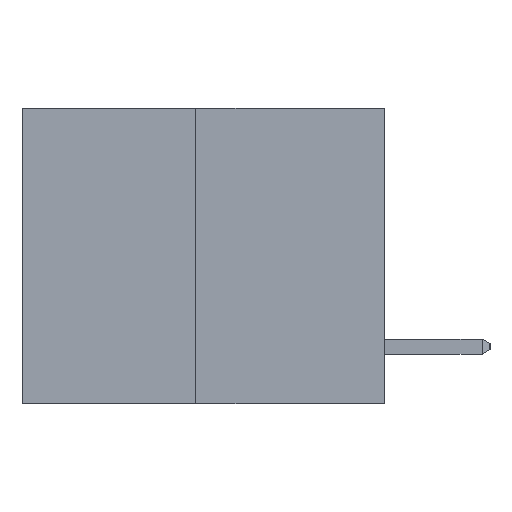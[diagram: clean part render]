
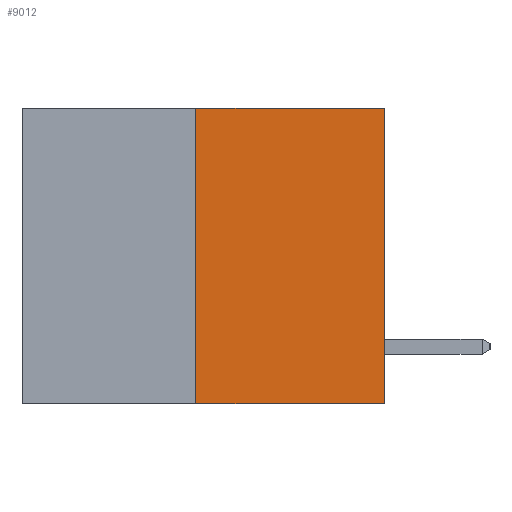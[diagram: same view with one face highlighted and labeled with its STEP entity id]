
A CAD part, left-side view. The second image highlights one B-rep face of the part: STEP entity #9012.
In plain terms, the highlighted planar face has unit normal (-1, 0, 0).
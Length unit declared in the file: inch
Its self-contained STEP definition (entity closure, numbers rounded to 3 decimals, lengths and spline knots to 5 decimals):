
#842 = EDGE_CURVE ( 'NONE', #2512, #4232, #8939, .T. ) ;
#925 = DIRECTION ( 'NONE',  ( 0., 0., 1. ) ) ;
#1031 = LINE ( 'NONE', #9667, #9418 ) ;
#1515 = CARTESIAN_POINT ( 'NONE',  ( 0., 0.312, 0. ) ) ;
#1947 = DIRECTION ( 'NONE',  ( 1., 0., 0. ) ) ;
#2512 = VERTEX_POINT ( 'NONE', #1515 ) ;
#2527 = ORIENTED_EDGE ( 'NONE', *, *, #4986, .F. ) ;
#2690 = CARTESIAN_POINT ( 'NONE',  ( 0., 0.6, -0.49 ) ) ;
#2900 = VECTOR ( 'NONE', #3539, 39.37008 ) ;
#3066 = ORIENTED_EDGE ( 'NONE', *, *, #842, .F. ) ;
#3245 = EDGE_CURVE ( 'NONE', #5120, #5028, #6477, .T. ) ;
#3539 = DIRECTION ( 'NONE',  ( 0., -1., 0. ) ) ;
#3736 = CARTESIAN_POINT ( 'NONE',  ( 0., 0., 0. ) ) ;
#3837 = ORIENTED_EDGE ( 'NONE', *, *, #8749, .T. ) ;
#3982 = VECTOR ( 'NONE', #925, 39.37008 ) ;
#4232 = VERTEX_POINT ( 'NONE', #3736 ) ;
#4310 = ORIENTED_EDGE ( 'NONE', *, *, #3245, .T. ) ;
#4333 = DIRECTION ( 'NONE',  ( 0., -1., 0. ) ) ;
#4986 = EDGE_CURVE ( 'NONE', #5120, #2512, #1031, .T. ) ;
#5028 = VERTEX_POINT ( 'NONE', #8066 ) ;
#5120 = VERTEX_POINT ( 'NONE', #8205 ) ;
#5175 = AXIS2_PLACEMENT_3D ( 'NONE', #6806, #1947, #9265 ) ;
#5258 = PLANE ( 'NONE',  #5175 ) ;
#5436 = DIRECTION ( 'NONE',  ( 0., 0., 1. ) ) ;
#5657 = CARTESIAN_POINT ( 'NONE',  ( 0., 0., 0. ) ) ;
#5740 = VECTOR ( 'NONE', #4333, 39.37008 ) ;
#6477 = LINE ( 'NONE', #2690, #2900 ) ;
#6806 = CARTESIAN_POINT ( 'NONE',  ( 0., 0.6, 0. ) ) ;
#8066 = CARTESIAN_POINT ( 'NONE',  ( 0., 0., -0.49 ) ) ;
#8205 = CARTESIAN_POINT ( 'NONE',  ( 0., 0.312, -0.49 ) ) ;
#8289 = EDGE_LOOP ( 'NONE', ( #2527, #4310, #3837, #3066 ) ) ;
#8327 = CARTESIAN_POINT ( 'NONE',  ( 0., 0.6, 0. ) ) ;
#8749 = EDGE_CURVE ( 'NONE', #5028, #4232, #9303, .T. ) ;
#8939 = LINE ( 'NONE', #8327, #5740 ) ;
#9012 = ADVANCED_FACE ( 'NONE', ( #10302 ), #5258, .F. ) ;
#9265 = DIRECTION ( 'NONE',  ( 0., 0., -1. ) ) ;
#9303 = LINE ( 'NONE', #5657, #3982 ) ;
#9418 = VECTOR ( 'NONE', #5436, 39.37008 ) ;
#9667 = CARTESIAN_POINT ( 'NONE',  ( 0., 0.312, -0.49 ) ) ;
#10302 = FACE_OUTER_BOUND ( 'NONE', #8289, .T. ) ;
